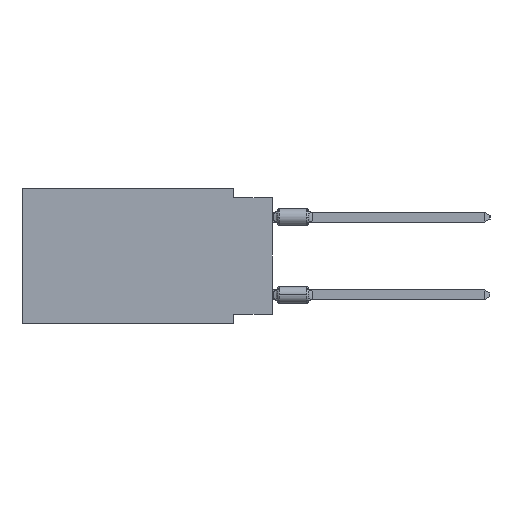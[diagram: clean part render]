
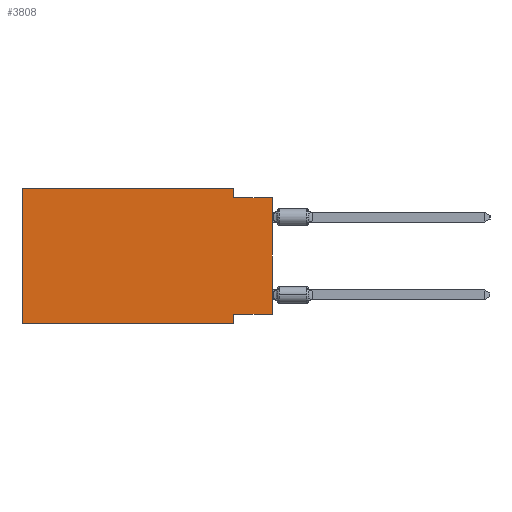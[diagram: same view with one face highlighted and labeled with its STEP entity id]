
A CAD part, left-side view. The second image highlights one B-rep face of the part: STEP entity #3808.
In plain terms, the highlighted planar face has unit normal (-1, 0, 0).
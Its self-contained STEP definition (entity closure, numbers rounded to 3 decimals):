
#392 = CARTESIAN_POINT ( 'NONE',  ( 0., 2.54, 0. ) ) ;
#1283 = DIRECTION ( 'NONE',  ( 0., -1., 0. ) ) ;
#3808 = ADVANCED_FACE ( 'NONE', ( #9409 ), #8404, .F. ) ;
#3843 = VERTEX_POINT ( 'NONE', #40054 ) ;
#5002 = LINE ( 'NONE', #57095, #45367 ) ;
#6370 = CARTESIAN_POINT ( 'NONE',  ( 0., 16.383, 0. ) ) ;
#8404 = PLANE ( 'NONE',  #15559 ) ;
#9301 = VERTEX_POINT ( 'NONE', #20361 ) ;
#9409 = FACE_OUTER_BOUND ( 'NONE', #47922, .T. ) ;
#10330 = EDGE_CURVE ( 'NONE', #29541, #11438, #5002, .T. ) ;
#10697 = VECTOR ( 'NONE', #60086, 1000. ) ;
#11438 = VERTEX_POINT ( 'NONE', #15706 ) ;
#13056 = CARTESIAN_POINT ( 'NONE',  ( 0., 0., 0. ) ) ;
#14343 = EDGE_CURVE ( 'NONE', #49305, #46734, #38276, .T. ) ;
#15559 = AXIS2_PLACEMENT_3D ( 'NONE', #19644, #54710, #65957 ) ;
#15594 = CARTESIAN_POINT ( 'NONE',  ( 0., 16.383, -8.89 ) ) ;
#15706 = CARTESIAN_POINT ( 'NONE',  ( 0., 2.54, -8.255 ) ) ;
#17040 = EDGE_CURVE ( 'NONE', #3843, #32263, #36137, .T. ) ;
#17688 = DIRECTION ( 'NONE',  ( 0., -1., 0. ) ) ;
#19644 = CARTESIAN_POINT ( 'NONE',  ( 0., 16.383, 0. ) ) ;
#20361 = CARTESIAN_POINT ( 'NONE',  ( 0., 2.54, -8.89 ) ) ;
#20843 = DIRECTION ( 'NONE',  ( 0., 0., -1. ) ) ;
#21094 = VECTOR ( 'NONE', #17688, 1000. ) ;
#21175 = EDGE_CURVE ( 'NONE', #32263, #25221, #65205, .T. ) ;
#22295 = LINE ( 'NONE', #13056, #42535 ) ;
#22827 = LINE ( 'NONE', #64350, #21094 ) ;
#24236 = VECTOR ( 'NONE', #31621, 1000. ) ;
#24934 = ORIENTED_EDGE ( 'NONE', *, *, #10330, .F. ) ;
#25221 = VERTEX_POINT ( 'NONE', #65941 ) ;
#26607 = ORIENTED_EDGE ( 'NONE', *, *, #29537, .T. ) ;
#26721 = LINE ( 'NONE', #57694, #55974 ) ;
#28073 = DIRECTION ( 'NONE',  ( 0., 0., 1. ) ) ;
#29537 = EDGE_CURVE ( 'NONE', #49305, #9301, #62259, .T. ) ;
#29541 = VERTEX_POINT ( 'NONE', #42804 ) ;
#31621 = DIRECTION ( 'NONE',  ( 0., 0., 1. ) ) ;
#31955 = CARTESIAN_POINT ( 'NONE',  ( 0., 16.383, 0. ) ) ;
#32263 = VERTEX_POINT ( 'NONE', #50986 ) ;
#33633 = ORIENTED_EDGE ( 'NONE', *, *, #59246, .F. ) ;
#33741 = ORIENTED_EDGE ( 'NONE', *, *, #17040, .F. ) ;
#35345 = VECTOR ( 'NONE', #20843, 1000. ) ;
#36137 = LINE ( 'NONE', #392, #35345 ) ;
#37198 = ORIENTED_EDGE ( 'NONE', *, *, #21175, .F. ) ;
#37595 = EDGE_CURVE ( 'NONE', #29541, #25221, #22295, .T. ) ;
#38276 = LINE ( 'NONE', #31955, #24236 ) ;
#39292 = CARTESIAN_POINT ( 'NONE',  ( 0., 0., -0.635 ) ) ;
#40054 = CARTESIAN_POINT ( 'NONE',  ( 0., 2.54, 0. ) ) ;
#42535 = VECTOR ( 'NONE', #28073, 1000. ) ;
#42804 = CARTESIAN_POINT ( 'NONE',  ( 0., 0., -8.255 ) ) ;
#44412 = CARTESIAN_POINT ( 'NONE',  ( 0., 16.383, -8.89 ) ) ;
#45149 = DIRECTION ( 'NONE',  ( 0., 1., 0. ) ) ;
#45367 = VECTOR ( 'NONE', #45149, 1000. ) ;
#46734 = VERTEX_POINT ( 'NONE', #6370 ) ;
#47922 = EDGE_LOOP ( 'NONE', ( #54076, #37198, #33741, #33633, #51906, #26607, #61139, #24934 ) ) ;
#49305 = VERTEX_POINT ( 'NONE', #44412 ) ;
#50986 = CARTESIAN_POINT ( 'NONE',  ( 0., 2.54, -0.635 ) ) ;
#51894 = EDGE_CURVE ( 'NONE', #11438, #9301, #26721, .T. ) ;
#51906 = ORIENTED_EDGE ( 'NONE', *, *, #14343, .F. ) ;
#54076 = ORIENTED_EDGE ( 'NONE', *, *, #37595, .T. ) ;
#54710 = DIRECTION ( 'NONE',  ( 1., 0., 0. ) ) ;
#55974 = VECTOR ( 'NONE', #62129, 1000. ) ;
#57095 = CARTESIAN_POINT ( 'NONE',  ( 0., 0., -8.255 ) ) ;
#57694 = CARTESIAN_POINT ( 'NONE',  ( 0., 2.54, -8.89 ) ) ;
#59246 = EDGE_CURVE ( 'NONE', #46734, #3843, #22827, .T. ) ;
#60086 = DIRECTION ( 'NONE',  ( 0., -1., 0. ) ) ;
#61139 = ORIENTED_EDGE ( 'NONE', *, *, #51894, .F. ) ;
#62129 = DIRECTION ( 'NONE',  ( 0., 0., -1. ) ) ;
#62259 = LINE ( 'NONE', #15594, #66167 ) ;
#64350 = CARTESIAN_POINT ( 'NONE',  ( 0., 16.383, 0. ) ) ;
#65205 = LINE ( 'NONE', #39292, #10697 ) ;
#65941 = CARTESIAN_POINT ( 'NONE',  ( 0., 0., -0.635 ) ) ;
#65957 = DIRECTION ( 'NONE',  ( 0., 0., -1. ) ) ;
#66167 = VECTOR ( 'NONE', #1283, 1000. ) ;
